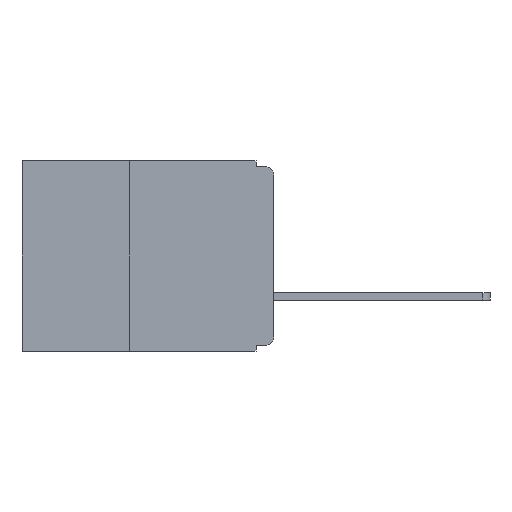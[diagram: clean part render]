
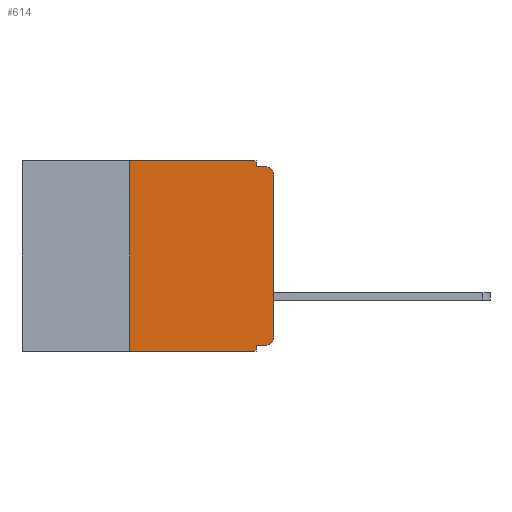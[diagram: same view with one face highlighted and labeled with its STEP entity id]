
A CAD part, left-side view. The second image highlights one B-rep face of the part: STEP entity #614.
In plain terms, the highlighted planar face has unit normal (-1, 0, 0).
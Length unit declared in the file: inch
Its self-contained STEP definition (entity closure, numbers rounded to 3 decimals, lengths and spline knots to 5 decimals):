
#264 = CARTESIAN_POINT ( 'NONE',  ( 0., 0.437, 0. ) ) ;
#614 = ADVANCED_FACE ( 'NONE', ( #5979 ), #6502, .F. ) ;
#745 = CARTESIAN_POINT ( 'NONE',  ( 0., 0., -0.305 ) ) ;
#1218 = DIRECTION ( 'NONE',  ( 0., -1., 0. ) ) ;
#1694 = CARTESIAN_POINT ( 'NONE',  ( 0., 0., -0.01 ) ) ;
#1981 = DIRECTION ( 'NONE',  ( -1., 0., 0. ) ) ;
#2113 = CARTESIAN_POINT ( 'NONE',  ( 0., 0.031, -0.01 ) ) ;
#2117 = VERTEX_POINT ( 'NONE', #745 ) ;
#2194 = DIRECTION ( 'NONE',  ( 0., 0., -1. ) ) ;
#2240 = CARTESIAN_POINT ( 'NONE',  ( 0., 0.015, -0.305 ) ) ;
#2241 = DIRECTION ( 'NONE',  ( 0., 0., 1. ) ) ;
#2279 = EDGE_CURVE ( 'NONE', #2117, #6179, #3085, .T. ) ;
#2325 = DIRECTION ( 'NONE',  ( 0., 1., 0. ) ) ;
#2353 = VECTOR ( 'NONE', #2325, 39.37008 ) ;
#2358 = CARTESIAN_POINT ( 'NONE',  ( 0., 0., -0.32 ) ) ;
#2729 = EDGE_CURVE ( 'NONE', #9970, #11015, #11669, .T. ) ;
#2739 = LINE ( 'NONE', #2358, #2353 ) ;
#2793 = VERTEX_POINT ( 'NONE', #13615 ) ;
#2976 = LINE ( 'NONE', #3197, #11584 ) ;
#3085 = LINE ( 'NONE', #14080, #8944 ) ;
#3121 = EDGE_CURVE ( 'NONE', #6357, #3739, #2739, .T. ) ;
#3197 = CARTESIAN_POINT ( 'NONE',  ( 0., 0.031, 0. ) ) ;
#3220 = DIRECTION ( 'NONE',  ( 0., -1., 0. ) ) ;
#3260 = EDGE_CURVE ( 'NONE', #6179, #11015, #7132, .T. ) ;
#3473 = CARTESIAN_POINT ( 'NONE',  ( 0., 0.25, -0.33 ) ) ;
#3624 = EDGE_CURVE ( 'NONE', #6357, #2117, #9420, .T. ) ;
#3739 = VERTEX_POINT ( 'NONE', #13471 ) ;
#4309 = VECTOR ( 'NONE', #1218, 39.37008 ) ;
#4499 = CARTESIAN_POINT ( 'NONE',  ( 0., 0.015, -0.32 ) ) ;
#4692 = LINE ( 'NONE', #13971, #12880 ) ;
#5393 = CARTESIAN_POINT ( 'NONE',  ( 0., 0.031, -0.33 ) ) ;
#5565 = VERTEX_POINT ( 'NONE', #7307 ) ;
#5901 = VECTOR ( 'NONE', #3220, 39.37008 ) ;
#5979 = FACE_OUTER_BOUND ( 'NONE', #11200, .T. ) ;
#6179 = VERTEX_POINT ( 'NONE', #9822 ) ;
#6348 = EDGE_CURVE ( 'NONE', #5565, #9970, #2976, .T. ) ;
#6357 = VERTEX_POINT ( 'NONE', #4499 ) ;
#6434 = EDGE_CURVE ( 'NONE', #10736, #2793, #4692, .T. ) ;
#6502 = PLANE ( 'NONE',  #12712 ) ;
#6510 = EDGE_CURVE ( 'NONE', #10736, #9150, #9690, .T. ) ;
#6542 = CARTESIAN_POINT ( 'NONE',  ( 0., 0.437, 0. ) ) ;
#6601 = DIRECTION ( 'NONE',  ( 1., 0., 0. ) ) ;
#6651 = DIRECTION ( 'NONE',  ( 0., 0., -1. ) ) ;
#6652 = EDGE_CURVE ( 'NONE', #3739, #9150, #7952, .T. ) ;
#7132 = CIRCLE ( 'NONE', #9162, 0.015 ) ;
#7307 = CARTESIAN_POINT ( 'NONE',  ( 0., 0.031, 0. ) ) ;
#7329 = CARTESIAN_POINT ( 'NONE',  ( 0., 0.031, -0.33 ) ) ;
#7566 = VECTOR ( 'NONE', #13408, 39.37008 ) ;
#7952 = LINE ( 'NONE', #7329, #7566 ) ;
#8276 = CARTESIAN_POINT ( 'NONE',  ( 0., 0.437, -0.33 ) ) ;
#8654 = AXIS2_PLACEMENT_3D ( 'NONE', #2240, #1981, #2194 ) ;
#8944 = VECTOR ( 'NONE', #13878, 39.37008 ) ;
#9150 = VERTEX_POINT ( 'NONE', #5393 ) ;
#9162 = AXIS2_PLACEMENT_3D ( 'NONE', #11953, #12046, #11848 ) ;
#9420 = CIRCLE ( 'NONE', #8654, 0.015 ) ;
#9630 = DIRECTION ( 'NONE',  ( 0., -1., 0. ) ) ;
#9690 = LINE ( 'NONE', #8276, #4309 ) ;
#9822 = CARTESIAN_POINT ( 'NONE',  ( 0., 0., -0.025 ) ) ;
#9862 = CARTESIAN_POINT ( 'NONE',  ( 0., 0.015, -0.01 ) ) ;
#9970 = VERTEX_POINT ( 'NONE', #2113 ) ;
#10574 = LINE ( 'NONE', #264, #12803 ) ;
#10736 = VERTEX_POINT ( 'NONE', #3473 ) ;
#11015 = VERTEX_POINT ( 'NONE', #9862 ) ;
#11200 = EDGE_LOOP ( 'NONE', ( #11806, #11817, #11884, #11995, #12092, #12169, #12297, #12663, #12692, #12976 ) ) ;
#11584 = VECTOR ( 'NONE', #12994, 39.37008 ) ;
#11669 = LINE ( 'NONE', #1694, #5901 ) ;
#11806 = ORIENTED_EDGE ( 'NONE', *, *, #2279, .T. ) ;
#11817 = ORIENTED_EDGE ( 'NONE', *, *, #3260, .T. ) ;
#11848 = DIRECTION ( 'NONE',  ( 0., 0., -1. ) ) ;
#11884 = ORIENTED_EDGE ( 'NONE', *, *, #2729, .F. ) ;
#11953 = CARTESIAN_POINT ( 'NONE',  ( 0., 0.015, -0.025 ) ) ;
#11995 = ORIENTED_EDGE ( 'NONE', *, *, #6348, .F. ) ;
#12046 = DIRECTION ( 'NONE',  ( -1., 0., 0. ) ) ;
#12092 = ORIENTED_EDGE ( 'NONE', *, *, #13901, .F. ) ;
#12169 = ORIENTED_EDGE ( 'NONE', *, *, #6434, .F. ) ;
#12297 = ORIENTED_EDGE ( 'NONE', *, *, #6510, .T. ) ;
#12663 = ORIENTED_EDGE ( 'NONE', *, *, #6652, .F. ) ;
#12692 = ORIENTED_EDGE ( 'NONE', *, *, #3121, .F. ) ;
#12712 = AXIS2_PLACEMENT_3D ( 'NONE', #6542, #6601, #6651 ) ;
#12803 = VECTOR ( 'NONE', #9630, 39.37008 ) ;
#12880 = VECTOR ( 'NONE', #2241, 39.37008 ) ;
#12976 = ORIENTED_EDGE ( 'NONE', *, *, #3624, .T. ) ;
#12994 = DIRECTION ( 'NONE',  ( 0., 0., -1. ) ) ;
#13408 = DIRECTION ( 'NONE',  ( 0., 0., -1. ) ) ;
#13471 = CARTESIAN_POINT ( 'NONE',  ( 0., 0.031, -0.32 ) ) ;
#13615 = CARTESIAN_POINT ( 'NONE',  ( 0., 0.25, 0. ) ) ;
#13878 = DIRECTION ( 'NONE',  ( 0., 0., 1. ) ) ;
#13901 = EDGE_CURVE ( 'NONE', #2793, #5565, #10574, .T. ) ;
#13971 = CARTESIAN_POINT ( 'NONE',  ( 0., 0.25, -0.33 ) ) ;
#14080 = CARTESIAN_POINT ( 'NONE',  ( 0., 0., 0. ) ) ;
